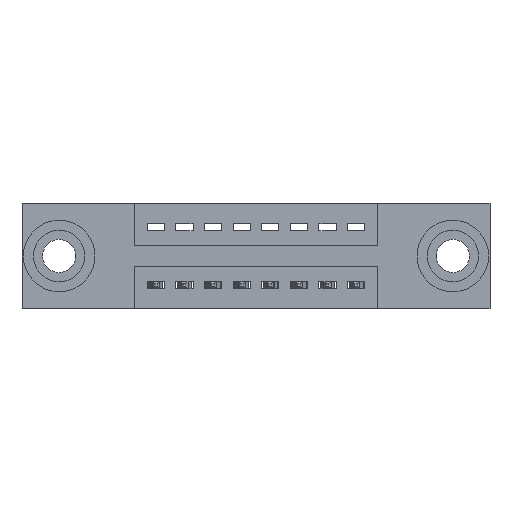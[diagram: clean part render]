
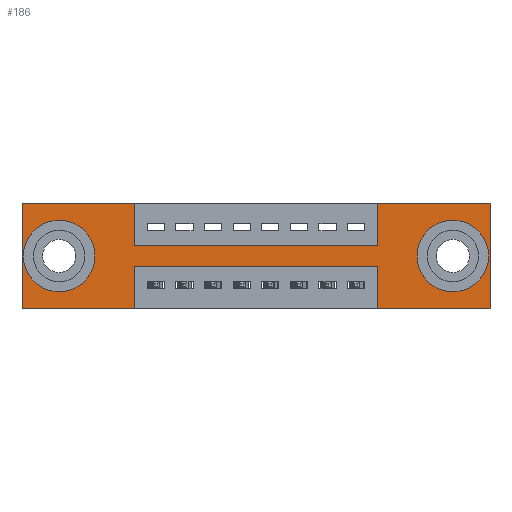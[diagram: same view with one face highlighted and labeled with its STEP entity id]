
A CAD part, front view. The second image highlights one B-rep face of the part: STEP entity #186.
In plain terms, the highlighted planar face has unit normal (0, -1, 0).
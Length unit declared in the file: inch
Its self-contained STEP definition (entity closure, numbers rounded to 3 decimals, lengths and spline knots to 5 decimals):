
#75 = VERTEX_POINT ( 'NONE', #7544 ) ;
#88 = CARTESIAN_POINT ( 'NONE',  ( 0.3925, 0., -0.37 ) ) ;
#186 = ADVANCED_FACE ( 'NONE', ( #7063, #330, #11038 ), #5085, .T. ) ;
#330 = FACE_BOUND ( 'NONE', #1762, .T. ) ;
#386 = CARTESIAN_POINT ( 'NONE',  ( 0.3925, 0., -0.37 ) ) ;
#407 = ORIENTED_EDGE ( 'NONE', *, *, #10249, .T. ) ;
#524 = DIRECTION ( 'NONE',  ( 0., 1., 0. ) ) ;
#601 = DIRECTION ( 'NONE',  ( 0., 0., 1. ) ) ;
#770 = VERTEX_POINT ( 'NONE', #4450 ) ;
#787 = CARTESIAN_POINT ( 'NONE',  ( 0.13, 0., -0.185 ) ) ;
#858 = VERTEX_POINT ( 'NONE', #3813 ) ;
#926 = EDGE_CURVE ( 'NONE', #6280, #6887, #3805, .T. ) ;
#933 = EDGE_CURVE ( 'NONE', #6425, #858, #3254, .T. ) ;
#1030 = VERTEX_POINT ( 'NONE', #4907 ) ;
#1064 = CARTESIAN_POINT ( 'NONE',  ( 0., 0., -0.37 ) ) ;
#1095 = EDGE_CURVE ( 'NONE', #3375, #3875, #2464, .T. ) ;
#1121 = DIRECTION ( 'NONE',  ( 0., 0., -1. ) ) ;
#1166 = CARTESIAN_POINT ( 'NONE',  ( 0., 0., 0. ) ) ;
#1310 = CARTESIAN_POINT ( 'NONE',  ( 1.2425, 0., 0. ) ) ;
#1320 = CARTESIAN_POINT ( 'NONE',  ( 1.505, 0., -0.263 ) ) ;
#1471 = DIRECTION ( 'NONE',  ( 0., -1., 0. ) ) ;
#1497 = EDGE_CURVE ( 'NONE', #3875, #9144, #8184, .T. ) ;
#1543 = CARTESIAN_POINT ( 'NONE',  ( 0., 0., -0.37 ) ) ;
#1571 = VECTOR ( 'NONE', #11284, 39.37008 ) ;
#1636 = CIRCLE ( 'NONE', #8130, 0.078 ) ;
#1674 = EDGE_LOOP ( 'NONE', ( #407, #5344 ) ) ;
#1723 = CARTESIAN_POINT ( 'NONE',  ( 0.13, 0., -0.185 ) ) ;
#1762 = EDGE_LOOP ( 'NONE', ( #7621, #5634 ) ) ;
#1971 = CARTESIAN_POINT ( 'NONE',  ( 1.2425, 0., -0.37 ) ) ;
#1986 = ORIENTED_EDGE ( 'NONE', *, *, #1095, .F. ) ;
#2017 = CARTESIAN_POINT ( 'NONE',  ( 0., 0., 0. ) ) ;
#2019 = VECTOR ( 'NONE', #11006, 39.37008 ) ;
#2136 = CARTESIAN_POINT ( 'NONE',  ( 1.2425, 0., -0.22 ) ) ;
#2361 = VERTEX_POINT ( 'NONE', #5894 ) ;
#2364 = CARTESIAN_POINT ( 'NONE',  ( 1.505, 0., -0.185 ) ) ;
#2464 = LINE ( 'NONE', #10214, #9107 ) ;
#2504 = CARTESIAN_POINT ( 'NONE',  ( 1.2425, 0., 0. ) ) ;
#2693 = CARTESIAN_POINT ( 'NONE',  ( 0., 0., -0.37 ) ) ;
#2726 = CIRCLE ( 'NONE', #7058, 0.078 ) ;
#2845 = AXIS2_PLACEMENT_3D ( 'NONE', #1543, #1471, #3466 ) ;
#2873 = DIRECTION ( 'NONE',  ( -1., 0., 0. ) ) ;
#2939 = EDGE_LOOP ( 'NONE', ( #7878, #3462, #3745, #8391, #10522, #4030, #6469, #10736, #1986, #4327, #6730, #8930 ) ) ;
#2983 = EDGE_CURVE ( 'NONE', #770, #5919, #6637, .T. ) ;
#3022 = VECTOR ( 'NONE', #6445, 39.37008 ) ;
#3106 = VECTOR ( 'NONE', #2873, 39.37008 ) ;
#3197 = EDGE_CURVE ( 'NONE', #5523, #75, #4368, .T. ) ;
#3254 = CIRCLE ( 'NONE', #6841, 0.078 ) ;
#3375 = VERTEX_POINT ( 'NONE', #10251 ) ;
#3462 = ORIENTED_EDGE ( 'NONE', *, *, #9045, .F. ) ;
#3466 = DIRECTION ( 'NONE',  ( 0., 0., -1. ) ) ;
#3745 = ORIENTED_EDGE ( 'NONE', *, *, #9465, .F. ) ;
#3753 = CARTESIAN_POINT ( 'NONE',  ( 0.13, 0., -0.107 ) ) ;
#3805 = LINE ( 'NONE', #4446, #10110 ) ;
#3813 = CARTESIAN_POINT ( 'NONE',  ( 0.13, 0., -0.263 ) ) ;
#3875 = VERTEX_POINT ( 'NONE', #9501 ) ;
#4030 = ORIENTED_EDGE ( 'NONE', *, *, #3197, .F. ) ;
#4327 = ORIENTED_EDGE ( 'NONE', *, *, #10213, .F. ) ;
#4368 = LINE ( 'NONE', #2017, #2019 ) ;
#4399 = LINE ( 'NONE', #7816, #8450 ) ;
#4446 = CARTESIAN_POINT ( 'NONE',  ( 0., 0., 0. ) ) ;
#4450 = CARTESIAN_POINT ( 'NONE',  ( 0.3925, 0., -0.22 ) ) ;
#4627 = VERTEX_POINT ( 'NONE', #1320 ) ;
#4702 = VECTOR ( 'NONE', #9969, 39.37008 ) ;
#4822 = CARTESIAN_POINT ( 'NONE',  ( 1.505, 0., -0.185 ) ) ;
#4884 = CIRCLE ( 'NONE', #4993, 0.078 ) ;
#4907 = CARTESIAN_POINT ( 'NONE',  ( 1.2425, 0., -0.37 ) ) ;
#4993 = AXIS2_PLACEMENT_3D ( 'NONE', #787, #524, #601 ) ;
#5085 = PLANE ( 'NONE',  #2845 ) ;
#5190 = EDGE_CURVE ( 'NONE', #858, #6425, #4884, .T. ) ;
#5344 = ORIENTED_EDGE ( 'NONE', *, *, #8611, .T. ) ;
#5421 = VECTOR ( 'NONE', #10586, 39.37008 ) ;
#5523 = VERTEX_POINT ( 'NONE', #2504 ) ;
#5634 = ORIENTED_EDGE ( 'NONE', *, *, #5190, .T. ) ;
#5750 = DIRECTION ( 'NONE',  ( 0., 0., -1. ) ) ;
#5894 = CARTESIAN_POINT ( 'NONE',  ( 1.635, 0., -0.37 ) ) ;
#5896 = VERTEX_POINT ( 'NONE', #2136 ) ;
#5919 = VERTEX_POINT ( 'NONE', #88 ) ;
#5965 = VECTOR ( 'NONE', #7623, 39.37008 ) ;
#6003 = DIRECTION ( 'NONE',  ( 0., 1., 0. ) ) ;
#6280 = VERTEX_POINT ( 'NONE', #2693 ) ;
#6331 = DIRECTION ( 'NONE',  ( 0., 0., 1. ) ) ;
#6425 = VERTEX_POINT ( 'NONE', #3753 ) ;
#6445 = DIRECTION ( 'NONE',  ( -1., 0., 0. ) ) ;
#6469 = ORIENTED_EDGE ( 'NONE', *, *, #9652, .F. ) ;
#6529 = DIRECTION ( 'NONE',  ( 0., 1., 0. ) ) ;
#6637 = LINE ( 'NONE', #386, #1571 ) ;
#6730 = ORIENTED_EDGE ( 'NONE', *, *, #926, .F. ) ;
#6841 = AXIS2_PLACEMENT_3D ( 'NONE', #1723, #6003, #6331 ) ;
#6887 = VERTEX_POINT ( 'NONE', #9637 ) ;
#6948 = VECTOR ( 'NONE', #11248, 39.37008 ) ;
#7058 = AXIS2_PLACEMENT_3D ( 'NONE', #4822, #10643, #5750 ) ;
#7063 = FACE_BOUND ( 'NONE', #1674, .T. ) ;
#7066 = LINE ( 'NONE', #1310, #4702 ) ;
#7191 = LINE ( 'NONE', #1971, #6948 ) ;
#7378 = CARTESIAN_POINT ( 'NONE',  ( 1.635, 0., 0. ) ) ;
#7417 = DIRECTION ( 'NONE',  ( 0., 0., -1. ) ) ;
#7478 = VERTEX_POINT ( 'NONE', #8686 ) ;
#7544 = CARTESIAN_POINT ( 'NONE',  ( 1.635, 0., 0. ) ) ;
#7621 = ORIENTED_EDGE ( 'NONE', *, *, #933, .T. ) ;
#7623 = DIRECTION ( 'NONE',  ( 1., 0., 0. ) ) ;
#7750 = EDGE_CURVE ( 'NONE', #75, #2361, #10407, .T. ) ;
#7816 = CARTESIAN_POINT ( 'NONE',  ( 0., 0., -0.37 ) ) ;
#7878 = ORIENTED_EDGE ( 'NONE', *, *, #2983, .F. ) ;
#8130 = AXIS2_PLACEMENT_3D ( 'NONE', #2364, #6529, #1121 ) ;
#8184 = LINE ( 'NONE', #9086, #5965 ) ;
#8252 = VECTOR ( 'NONE', #7417, 39.37008 ) ;
#8391 = ORIENTED_EDGE ( 'NONE', *, *, #10568, .F. ) ;
#8450 = VECTOR ( 'NONE', #9459, 39.37008 ) ;
#8611 = EDGE_CURVE ( 'NONE', #4627, #7478, #1636, .T. ) ;
#8686 = CARTESIAN_POINT ( 'NONE',  ( 1.505, 0., -0.107 ) ) ;
#8930 = ORIENTED_EDGE ( 'NONE', *, *, #10858, .F. ) ;
#9045 = EDGE_CURVE ( 'NONE', #5896, #770, #9886, .T. ) ;
#9086 = CARTESIAN_POINT ( 'NONE',  ( 0.3925, 0., -0.15 ) ) ;
#9107 = VECTOR ( 'NONE', #10246, 39.37008 ) ;
#9144 = VERTEX_POINT ( 'NONE', #10022 ) ;
#9459 = DIRECTION ( 'NONE',  ( -1., 0., 0. ) ) ;
#9465 = EDGE_CURVE ( 'NONE', #1030, #5896, #7191, .T. ) ;
#9501 = CARTESIAN_POINT ( 'NONE',  ( 0.3925, 0., -0.15 ) ) ;
#9637 = CARTESIAN_POINT ( 'NONE',  ( 0., 0., 0. ) ) ;
#9652 = EDGE_CURVE ( 'NONE', #9144, #5523, #7066, .T. ) ;
#9718 = CARTESIAN_POINT ( 'NONE',  ( 0.3925, 0., -0.22 ) ) ;
#9859 = LINE ( 'NONE', #1166, #5421 ) ;
#9886 = LINE ( 'NONE', #9718, #3022 ) ;
#9965 = LINE ( 'NONE', #1064, #3106 ) ;
#9969 = DIRECTION ( 'NONE',  ( 0., 0., 1. ) ) ;
#10022 = CARTESIAN_POINT ( 'NONE',  ( 1.2425, 0., -0.15 ) ) ;
#10110 = VECTOR ( 'NONE', #10364, 39.37008 ) ;
#10213 = EDGE_CURVE ( 'NONE', #6887, #3375, #9859, .T. ) ;
#10214 = CARTESIAN_POINT ( 'NONE',  ( 0.3925, 0., 0. ) ) ;
#10246 = DIRECTION ( 'NONE',  ( 0., 0., -1. ) ) ;
#10249 = EDGE_CURVE ( 'NONE', #7478, #4627, #2726, .T. ) ;
#10251 = CARTESIAN_POINT ( 'NONE',  ( 0.3925, 0., 0. ) ) ;
#10364 = DIRECTION ( 'NONE',  ( 0., 0., 1. ) ) ;
#10407 = LINE ( 'NONE', #7378, #8252 ) ;
#10522 = ORIENTED_EDGE ( 'NONE', *, *, #7750, .F. ) ;
#10568 = EDGE_CURVE ( 'NONE', #2361, #1030, #4399, .T. ) ;
#10586 = DIRECTION ( 'NONE',  ( 1., 0., 0. ) ) ;
#10643 = DIRECTION ( 'NONE',  ( 0., 1., 0. ) ) ;
#10736 = ORIENTED_EDGE ( 'NONE', *, *, #1497, .F. ) ;
#10858 = EDGE_CURVE ( 'NONE', #5919, #6280, #9965, .T. ) ;
#11006 = DIRECTION ( 'NONE',  ( 1., 0., 0. ) ) ;
#11038 = FACE_OUTER_BOUND ( 'NONE', #2939, .T. ) ;
#11248 = DIRECTION ( 'NONE',  ( 0., 0., 1. ) ) ;
#11284 = DIRECTION ( 'NONE',  ( 0., 0., -1. ) ) ;
